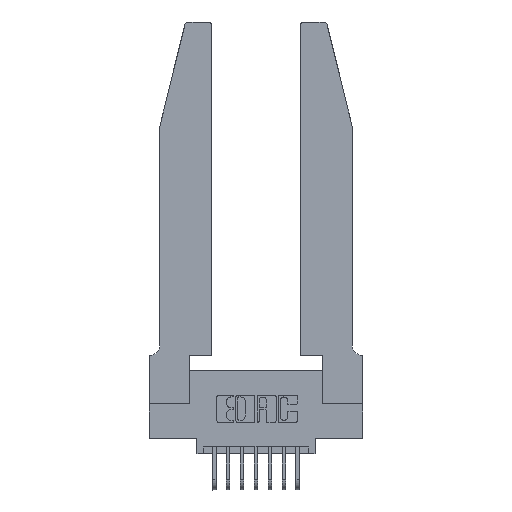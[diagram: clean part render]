
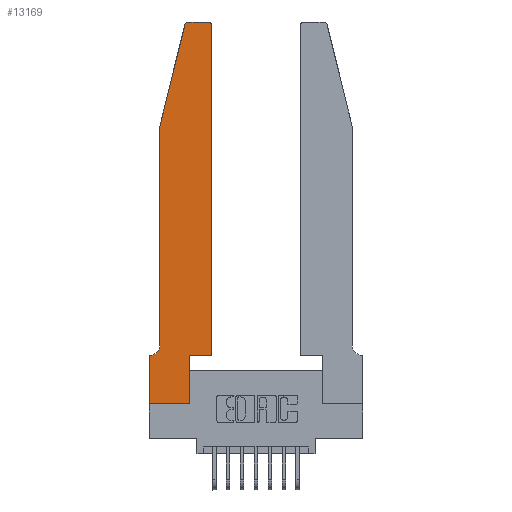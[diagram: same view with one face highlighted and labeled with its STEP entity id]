
A CAD part, top view. The second image highlights one B-rep face of the part: STEP entity #13169.
In plain terms, the highlighted planar face has unit normal (0, 0, 1).
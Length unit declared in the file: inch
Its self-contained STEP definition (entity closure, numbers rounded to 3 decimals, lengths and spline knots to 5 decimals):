
#183 = VERTEX_POINT ( 'NONE', #9756 ) ;
#190 = EDGE_CURVE ( 'NONE', #8183, #12222, #9372, .T. ) ;
#295 = EDGE_LOOP ( 'NONE', ( #2774, #6542, #11588, #9884, #3255, #10279, #12232, #12066, #1329, #9072, #8737, #13873 ) ) ;
#381 = VECTOR ( 'NONE', #9920, 39.37008 ) ;
#499 = EDGE_CURVE ( 'NONE', #7083, #10519, #11836, .T. ) ;
#553 = CARTESIAN_POINT ( 'NONE',  ( 0.4205, 2.75, 0.37 ) ) ;
#695 = EDGE_CURVE ( 'NONE', #6570, #13409, #14659, .T. ) ;
#946 = VECTOR ( 'NONE', #10196, 39.37008 ) ;
#1027 = EDGE_CURVE ( 'NONE', #12540, #1224, #13398, .T. ) ;
#1224 = VERTEX_POINT ( 'NONE', #7160 ) ;
#1329 = ORIENTED_EDGE ( 'NONE', *, *, #190, .T. ) ;
#1419 = EDGE_CURVE ( 'NONE', #10519, #4988, #9363, .T. ) ;
#1451 = AXIS2_PLACEMENT_3D ( 'NONE', #4174, #12271, #5384 ) ;
#1589 = DIRECTION ( 'NONE',  ( 1., 0., 0. ) ) ;
#2774 = ORIENTED_EDGE ( 'NONE', *, *, #14745, .T. ) ;
#2864 = VECTOR ( 'NONE', #12060, 39.37008 ) ;
#3255 = ORIENTED_EDGE ( 'NONE', *, *, #14227, .T. ) ;
#3818 = DIRECTION ( 'NONE',  ( -1., 0., 0. ) ) ;
#3946 = CARTESIAN_POINT ( 'NONE',  ( 0., 0.35, 0.37 ) ) ;
#4174 = CARTESIAN_POINT ( 'NONE',  ( 0.0055, 0.42, 0.37 ) ) ;
#4226 = VECTOR ( 'NONE', #13850, 39.37008 ) ;
#4654 = CARTESIAN_POINT ( 'NONE',  ( 0.2865, 0.35, 0.37 ) ) ;
#4700 = EDGE_CURVE ( 'NONE', #13409, #8183, #14426, .T. ) ;
#4928 = VERTEX_POINT ( 'NONE', #10290 ) ;
#4988 = VERTEX_POINT ( 'NONE', #553 ) ;
#5158 = CARTESIAN_POINT ( 'NONE',  ( 0., 0., 0.37 ) ) ;
#5227 = CIRCLE ( 'NONE', #1451, 0.07 ) ;
#5384 = DIRECTION ( 'NONE',  ( -1., 0., 0. ) ) ;
#5638 = CARTESIAN_POINT ( 'NONE',  ( 0., 0.35, 0.37 ) ) ;
#5658 = CARTESIAN_POINT ( 'NONE',  ( 0.4505, 2.72, 0.37 ) ) ;
#5688 = DIRECTION ( 'NONE',  ( 0., 0., 1. ) ) ;
#5875 = CARTESIAN_POINT ( 'NONE',  ( 0.2865, 0., 0.37 ) ) ;
#5999 = FACE_OUTER_BOUND ( 'NONE', #295, .T. ) ;
#6429 = LINE ( 'NONE', #14200, #12533 ) ;
#6542 = ORIENTED_EDGE ( 'NONE', *, *, #13188, .T. ) ;
#6570 = VERTEX_POINT ( 'NONE', #3946 ) ;
#6828 = DIRECTION ( 'NONE',  ( 1., 0., 0. ) ) ;
#7083 = VERTEX_POINT ( 'NONE', #12982 ) ;
#7160 = CARTESIAN_POINT ( 'NONE',  ( 0.0755, 2., 0.37 ) ) ;
#7484 = VERTEX_POINT ( 'NONE', #8132 ) ;
#8132 = CARTESIAN_POINT ( 'NONE',  ( 0.284, 2.75, 0.37 ) ) ;
#8183 = VERTEX_POINT ( 'NONE', #5875 ) ;
#8444 = VECTOR ( 'NONE', #10589, 39.37008 ) ;
#8692 = EDGE_CURVE ( 'NONE', #1224, #4928, #11852, .T. ) ;
#8737 = ORIENTED_EDGE ( 'NONE', *, *, #499, .T. ) ;
#8761 = EDGE_CURVE ( 'NONE', #12222, #7083, #10447, .T. ) ;
#8879 = DIRECTION ( 'NONE',  ( 0., 0., 1. ) ) ;
#8984 = CARTESIAN_POINT ( 'NONE',  ( 0.4205, 2.72, 0.37 ) ) ;
#9051 = CARTESIAN_POINT ( 'NONE',  ( 0.2605, 2.75, 0.37 ) ) ;
#9072 = ORIENTED_EDGE ( 'NONE', *, *, #8761, .T. ) ;
#9363 = CIRCLE ( 'NONE', #12613, 0.03 ) ;
#9372 = LINE ( 'NONE', #9394, #381 ) ;
#9394 = CARTESIAN_POINT ( 'NONE',  ( 0.2865, 0.35, 0.37 ) ) ;
#9756 = CARTESIAN_POINT ( 'NONE',  ( 0.0055, 0.35, 0.37 ) ) ;
#9884 = ORIENTED_EDGE ( 'NONE', *, *, #8692, .T. ) ;
#9920 = DIRECTION ( 'NONE',  ( 0., 1., 0. ) ) ;
#10094 = EDGE_CURVE ( 'NONE', #183, #6570, #6429, .T. ) ;
#10196 = DIRECTION ( 'NONE',  ( -1., 0., 0. ) ) ;
#10279 = ORIENTED_EDGE ( 'NONE', *, *, #10094, .T. ) ;
#10290 = CARTESIAN_POINT ( 'NONE',  ( 0.0755, 0.42, 0.37 ) ) ;
#10363 = CARTESIAN_POINT ( 'NONE',  ( 0.0755, 2., 0.37 ) ) ;
#10416 = VECTOR ( 'NONE', #10866, 39.37008 ) ;
#10447 = LINE ( 'NONE', #10454, #4226 ) ;
#10454 = CARTESIAN_POINT ( 'NONE',  ( 0.4505, 0.35, 0.37 ) ) ;
#10519 = VERTEX_POINT ( 'NONE', #5658 ) ;
#10589 = DIRECTION ( 'NONE',  ( 0., 1., 0. ) ) ;
#10866 = DIRECTION ( 'NONE',  ( -0.239, -0.971, 0. ) ) ;
#11307 = VECTOR ( 'NONE', #13027, 39.37008 ) ;
#11511 = VECTOR ( 'NONE', #13709, 39.37008 ) ;
#11588 = ORIENTED_EDGE ( 'NONE', *, *, #1027, .T. ) ;
#11612 = CARTESIAN_POINT ( 'NONE',  ( 0.0755, 2., 0.37 ) ) ;
#11751 = CIRCLE ( 'NONE', #14138, 0.03 ) ;
#11836 = LINE ( 'NONE', #12616, #8444 ) ;
#11852 = LINE ( 'NONE', #10363, #11511 ) ;
#12060 = DIRECTION ( 'NONE',  ( 1., 0., 0. ) ) ;
#12066 = ORIENTED_EDGE ( 'NONE', *, *, #4700, .T. ) ;
#12222 = VERTEX_POINT ( 'NONE', #4654 ) ;
#12232 = ORIENTED_EDGE ( 'NONE', *, *, #695, .T. ) ;
#12271 = DIRECTION ( 'NONE',  ( 0., 0., -1. ) ) ;
#12518 = PLANE ( 'NONE',  #14896 ) ;
#12533 = VECTOR ( 'NONE', #3818, 39.37008 ) ;
#12540 = VERTEX_POINT ( 'NONE', #14401 ) ;
#12563 = CARTESIAN_POINT ( 'NONE',  ( 0.284, 2.72, 0.37 ) ) ;
#12613 = AXIS2_PLACEMENT_3D ( 'NONE', #8984, #8879, #1589 ) ;
#12616 = CARTESIAN_POINT ( 'NONE',  ( 0.4505, 0.35, 0.37 ) ) ;
#12982 = CARTESIAN_POINT ( 'NONE',  ( 0.4505, 0.35, 0.37 ) ) ;
#12984 = CARTESIAN_POINT ( 'NONE',  ( 0., 0., 0.37 ) ) ;
#12993 = CARTESIAN_POINT ( 'NONE',  ( 0., 0., 0.37 ) ) ;
#13027 = DIRECTION ( 'NONE',  ( 0., -1., 0. ) ) ;
#13169 = ADVANCED_FACE ( 'NONE', ( #5999 ), #12518, .T. ) ;
#13188 = EDGE_CURVE ( 'NONE', #7484, #12540, #11751, .T. ) ;
#13398 = LINE ( 'NONE', #11612, #10416 ) ;
#13409 = VERTEX_POINT ( 'NONE', #12993 ) ;
#13640 = DIRECTION ( 'NONE',  ( 0., 0., 1. ) ) ;
#13647 = LINE ( 'NONE', #9051, #946 ) ;
#13695 = DIRECTION ( 'NONE',  ( 1., 0., 0. ) ) ;
#13709 = DIRECTION ( 'NONE',  ( 0., -1., 0. ) ) ;
#13850 = DIRECTION ( 'NONE',  ( 1., 0., 0. ) ) ;
#13873 = ORIENTED_EDGE ( 'NONE', *, *, #1419, .T. ) ;
#14138 = AXIS2_PLACEMENT_3D ( 'NONE', #12563, #5688, #13695 ) ;
#14200 = CARTESIAN_POINT ( 'NONE',  ( 0.0755, 0.35, 0.37 ) ) ;
#14227 = EDGE_CURVE ( 'NONE', #4928, #183, #5227, .T. ) ;
#14401 = CARTESIAN_POINT ( 'NONE',  ( 0.25487, 2.72718, 0.37 ) ) ;
#14426 = LINE ( 'NONE', #5158, #2864 ) ;
#14659 = LINE ( 'NONE', #12984, #11307 ) ;
#14745 = EDGE_CURVE ( 'NONE', #4988, #7484, #13647, .T. ) ;
#14896 = AXIS2_PLACEMENT_3D ( 'NONE', #5638, #13640, #6828 ) ;
